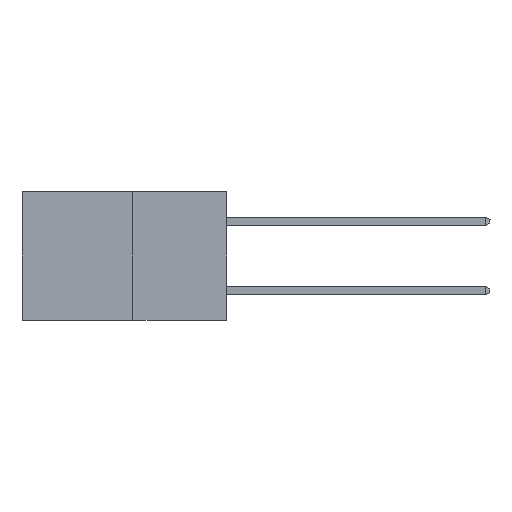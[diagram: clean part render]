
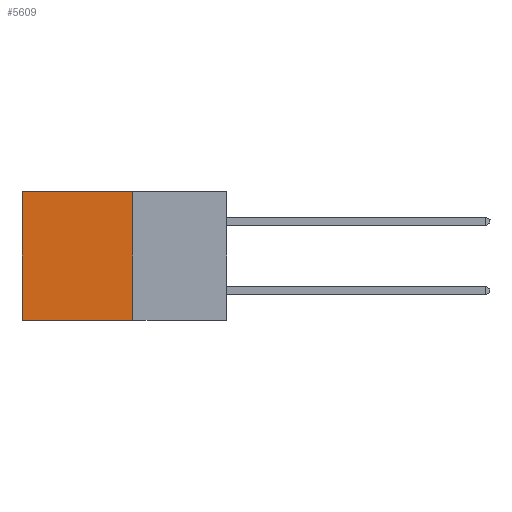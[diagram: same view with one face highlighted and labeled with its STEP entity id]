
A CAD part, left-side view. The second image highlights one B-rep face of the part: STEP entity #5609.
In plain terms, the highlighted planar face has unit normal (-1, 0, 0).
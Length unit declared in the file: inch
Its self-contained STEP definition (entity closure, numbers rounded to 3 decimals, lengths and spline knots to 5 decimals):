
#1195 = CARTESIAN_POINT ( 'NONE',  ( 0.277, 0.27, -0.37 ) ) ;
#1241 = LINE ( 'NONE', #1195, #12549 ) ;
#1500 = CARTESIAN_POINT ( 'NONE',  ( 0.277, 0.59, 0. ) ) ;
#2022 = CARTESIAN_POINT ( 'NONE',  ( 0.277, 0.27, 0. ) ) ;
#2694 = ORIENTED_EDGE ( 'NONE', *, *, #10748, .T. ) ;
#2818 = AXIS2_PLACEMENT_3D ( 'NONE', #9236, #11014, #10888 ) ;
#3055 = ORIENTED_EDGE ( 'NONE', *, *, #10790, .T. ) ;
#3762 = DIRECTION ( 'NONE',  ( 0., 1., 0. ) ) ;
#3857 = CARTESIAN_POINT ( 'NONE',  ( 0.277, 0.27, 0. ) ) ;
#4038 = CARTESIAN_POINT ( 'NONE',  ( 0.277, 0.59, -0.37 ) ) ;
#4056 = DIRECTION ( 'NONE',  ( 0., 0., -1. ) ) ;
#4147 = EDGE_CURVE ( 'NONE', #6946, #10614, #8882, .T. ) ;
#4303 = VERTEX_POINT ( 'NONE', #1500 ) ;
#4538 = EDGE_CURVE ( 'NONE', #10614, #8840, #1241, .T. ) ;
#4659 = ORIENTED_EDGE ( 'NONE', *, *, #4147, .F. ) ;
#4703 = LINE ( 'NONE', #3857, #10704 ) ;
#5534 = CARTESIAN_POINT ( 'NONE',  ( 0.277, 0.27, -0.37 ) ) ;
#5609 = ADVANCED_FACE ( 'NONE', ( #13565 ), #9421, .F. ) ;
#5716 = ORIENTED_EDGE ( 'NONE', *, *, #4538, .F. ) ;
#5769 = LINE ( 'NONE', #4038, #8081 ) ;
#6221 = VECTOR ( 'NONE', #12172, 39.37008 ) ;
#6946 = VERTEX_POINT ( 'NONE', #2022 ) ;
#8081 = VECTOR ( 'NONE', #4056, 39.37008 ) ;
#8710 = CARTESIAN_POINT ( 'NONE',  ( 0.277, 0.59, -0.37 ) ) ;
#8840 = VERTEX_POINT ( 'NONE', #8710 ) ;
#8882 = LINE ( 'NONE', #12325, #6221 ) ;
#9236 = CARTESIAN_POINT ( 'NONE',  ( 0.277, 0.27, -0.37 ) ) ;
#9421 = PLANE ( 'NONE',  #2818 ) ;
#10614 = VERTEX_POINT ( 'NONE', #5534 ) ;
#10704 = VECTOR ( 'NONE', #3762, 39.37008 ) ;
#10748 = EDGE_CURVE ( 'NONE', #4303, #8840, #5769, .T. ) ;
#10790 = EDGE_CURVE ( 'NONE', #6946, #4303, #4703, .T. ) ;
#10888 = DIRECTION ( 'NONE',  ( 0., 0., -1. ) ) ;
#10985 = EDGE_LOOP ( 'NONE', ( #2694, #5716, #4659, #3055 ) ) ;
#11014 = DIRECTION ( 'NONE',  ( 1., 0., 0. ) ) ;
#12172 = DIRECTION ( 'NONE',  ( 0., 0., -1. ) ) ;
#12325 = CARTESIAN_POINT ( 'NONE',  ( 0.277, 0.27, -0.37 ) ) ;
#12549 = VECTOR ( 'NONE', #13476, 39.37008 ) ;
#13476 = DIRECTION ( 'NONE',  ( 0., 1., 0. ) ) ;
#13565 = FACE_OUTER_BOUND ( 'NONE', #10985, .T. ) ;
